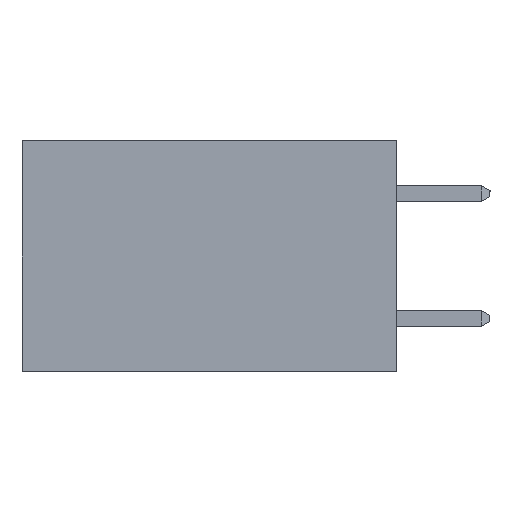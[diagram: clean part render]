
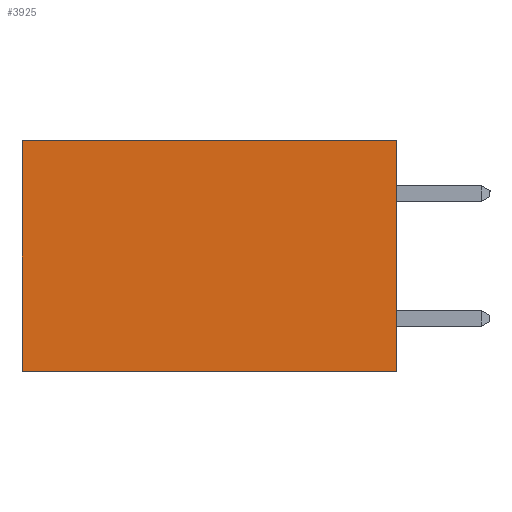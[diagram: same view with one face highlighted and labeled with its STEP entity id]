
A CAD part, left-side view. The second image highlights one B-rep face of the part: STEP entity #3925.
In plain terms, the highlighted planar face has unit normal (-1, 0, 0).
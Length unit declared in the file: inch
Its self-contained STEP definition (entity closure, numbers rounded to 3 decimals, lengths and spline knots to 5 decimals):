
#16 = LINE ( 'NONE', #4395, #1154 ) ;
#210 = ORIENTED_EDGE ( 'NONE', *, *, #4465, .T. ) ;
#319 = LINE ( 'NONE', #8848, #3798 ) ;
#746 = CARTESIAN_POINT ( 'NONE',  ( 0.2615, 0., -0.37 ) ) ;
#1154 = VECTOR ( 'NONE', #5748, 39.37008 ) ;
#1421 = EDGE_CURVE ( 'NONE', #2356, #8699, #1697, .T. ) ;
#1697 = LINE ( 'NONE', #5917, #6740 ) ;
#2165 = DIRECTION ( 'NONE',  ( 1., 0., 0. ) ) ;
#2356 = VERTEX_POINT ( 'NONE', #8383 ) ;
#2455 = ORIENTED_EDGE ( 'NONE', *, *, #2574, .F. ) ;
#2574 = EDGE_CURVE ( 'NONE', #3325, #2356, #319, .T. ) ;
#2892 = VECTOR ( 'NONE', #5435, 39.37008 ) ;
#3037 = VERTEX_POINT ( 'NONE', #3850 ) ;
#3046 = DIRECTION ( 'NONE',  ( 0., 0., -1. ) ) ;
#3126 = EDGE_LOOP ( 'NONE', ( #6596, #6899, #2455, #210 ) ) ;
#3141 = DIRECTION ( 'NONE',  ( 0., 1., 0. ) ) ;
#3325 = VERTEX_POINT ( 'NONE', #8073 ) ;
#3798 = VECTOR ( 'NONE', #3046, 39.37008 ) ;
#3850 = CARTESIAN_POINT ( 'NONE',  ( 0.2615, 0.6, 0. ) ) ;
#3925 = ADVANCED_FACE ( 'NONE', ( #4369 ), #5818, .F. ) ;
#4369 = FACE_OUTER_BOUND ( 'NONE', #3126, .T. ) ;
#4395 = CARTESIAN_POINT ( 'NONE',  ( 0.2615, 0., 0. ) ) ;
#4465 = EDGE_CURVE ( 'NONE', #3325, #3037, #16, .T. ) ;
#5435 = DIRECTION ( 'NONE',  ( 0., 0., -1. ) ) ;
#5503 = CARTESIAN_POINT ( 'NONE',  ( 0.2615, 0.6, -0.37 ) ) ;
#5748 = DIRECTION ( 'NONE',  ( 0., 1., 0. ) ) ;
#5818 = PLANE ( 'NONE',  #9198 ) ;
#5917 = CARTESIAN_POINT ( 'NONE',  ( 0.2615, 0., -0.37 ) ) ;
#6574 = DIRECTION ( 'NONE',  ( 0., 0., -1. ) ) ;
#6596 = ORIENTED_EDGE ( 'NONE', *, *, #6901, .T. ) ;
#6740 = VECTOR ( 'NONE', #3141, 39.37008 ) ;
#6899 = ORIENTED_EDGE ( 'NONE', *, *, #1421, .F. ) ;
#6901 = EDGE_CURVE ( 'NONE', #3037, #8699, #9271, .T. ) ;
#7081 = CARTESIAN_POINT ( 'NONE',  ( 0.2615, 0.6, -0.37 ) ) ;
#8073 = CARTESIAN_POINT ( 'NONE',  ( 0.2615, 0., 0. ) ) ;
#8383 = CARTESIAN_POINT ( 'NONE',  ( 0.2615, 0., -0.37 ) ) ;
#8699 = VERTEX_POINT ( 'NONE', #5503 ) ;
#8848 = CARTESIAN_POINT ( 'NONE',  ( 0.2615, 0., -0.37 ) ) ;
#9198 = AXIS2_PLACEMENT_3D ( 'NONE', #746, #2165, #6574 ) ;
#9271 = LINE ( 'NONE', #7081, #2892 ) ;
